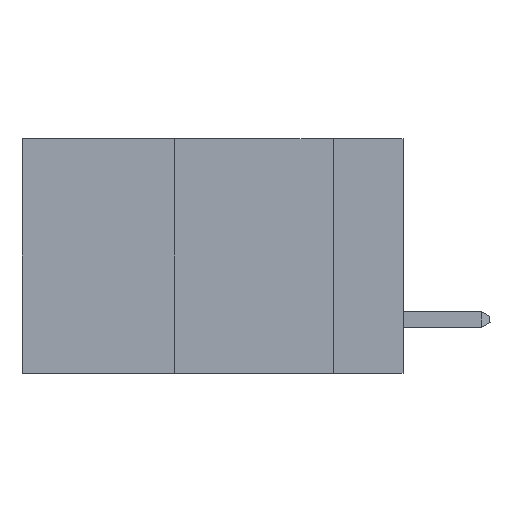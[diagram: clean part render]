
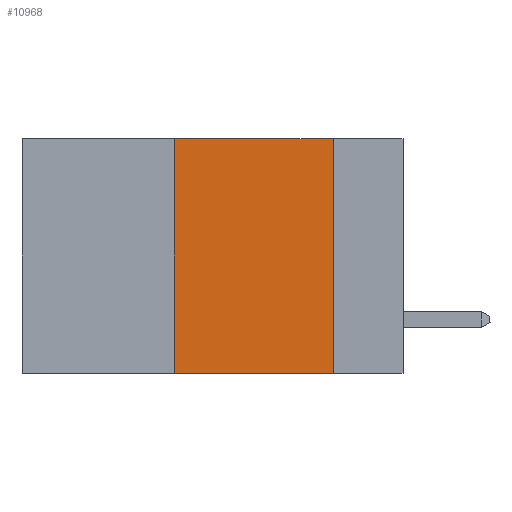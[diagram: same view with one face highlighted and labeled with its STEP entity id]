
A CAD part, left-side view. The second image highlights one B-rep face of the part: STEP entity #10968.
In plain terms, the highlighted planar face has unit normal (-1, 0, 0).
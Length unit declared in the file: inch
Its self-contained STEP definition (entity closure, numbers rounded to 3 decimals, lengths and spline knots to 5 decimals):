
#108 = VERTEX_POINT ( 'NONE', #4074 ) ;
#146 = ORIENTED_EDGE ( 'NONE', *, *, #8771, .F. ) ;
#359 = LINE ( 'NONE', #11974, #10374 ) ;
#577 = VERTEX_POINT ( 'NONE', #1409 ) ;
#967 = VERTEX_POINT ( 'NONE', #11625 ) ;
#1320 = DIRECTION ( 'NONE',  ( 0., 0., 1. ) ) ;
#1409 = CARTESIAN_POINT ( 'NONE',  ( 0., 0.36, -0.37 ) ) ;
#1552 = DIRECTION ( 'NONE',  ( 1., 0., 0. ) ) ;
#1871 = EDGE_CURVE ( 'NONE', #967, #2335, #2359, .T. ) ;
#2335 = VERTEX_POINT ( 'NONE', #10647 ) ;
#2359 = LINE ( 'NONE', #12031, #4765 ) ;
#2593 = PLANE ( 'NONE',  #8887 ) ;
#2666 = DIRECTION ( 'NONE',  ( 0., 0., -1. ) ) ;
#3282 = DIRECTION ( 'NONE',  ( 0., -1., 0. ) ) ;
#3410 = DIRECTION ( 'NONE',  ( 0., -1., 0. ) ) ;
#3802 = DIRECTION ( 'NONE',  ( 0., 0., -1. ) ) ;
#4074 = CARTESIAN_POINT ( 'NONE',  ( 0., 0.11, -0.37 ) ) ;
#4765 = VECTOR ( 'NONE', #3410, 39.37008 ) ;
#4785 = ORIENTED_EDGE ( 'NONE', *, *, #1871, .F. ) ;
#4889 = EDGE_LOOP ( 'NONE', ( #9996, #4785, #146, #11959 ) ) ;
#7526 = VECTOR ( 'NONE', #3802, 39.37008 ) ;
#7557 = EDGE_CURVE ( 'NONE', #2335, #108, #12056, .T. ) ;
#7700 = CARTESIAN_POINT ( 'NONE',  ( 0., 0.11, 0. ) ) ;
#8771 = EDGE_CURVE ( 'NONE', #577, #967, #359, .T. ) ;
#8887 = AXIS2_PLACEMENT_3D ( 'NONE', #10412, #1552, #2666 ) ;
#9221 = FACE_OUTER_BOUND ( 'NONE', #4889, .T. ) ;
#9653 = LINE ( 'NONE', #10148, #12355 ) ;
#9996 = ORIENTED_EDGE ( 'NONE', *, *, #7557, .F. ) ;
#10148 = CARTESIAN_POINT ( 'NONE',  ( 0., 0.6, -0.37 ) ) ;
#10374 = VECTOR ( 'NONE', #1320, 39.37008 ) ;
#10412 = CARTESIAN_POINT ( 'NONE',  ( 0., 0.6, 0. ) ) ;
#10647 = CARTESIAN_POINT ( 'NONE',  ( 0., 0.11, 0. ) ) ;
#10968 = ADVANCED_FACE ( 'NONE', ( #9221 ), #2593, .F. ) ;
#11625 = CARTESIAN_POINT ( 'NONE',  ( 0., 0.36, 0. ) ) ;
#11776 = EDGE_CURVE ( 'NONE', #577, #108, #9653, .T. ) ;
#11959 = ORIENTED_EDGE ( 'NONE', *, *, #11776, .T. ) ;
#11974 = CARTESIAN_POINT ( 'NONE',  ( 0., 0.36, 0. ) ) ;
#12031 = CARTESIAN_POINT ( 'NONE',  ( 0., 0.6, 0. ) ) ;
#12056 = LINE ( 'NONE', #7700, #7526 ) ;
#12355 = VECTOR ( 'NONE', #3282, 39.37008 ) ;
